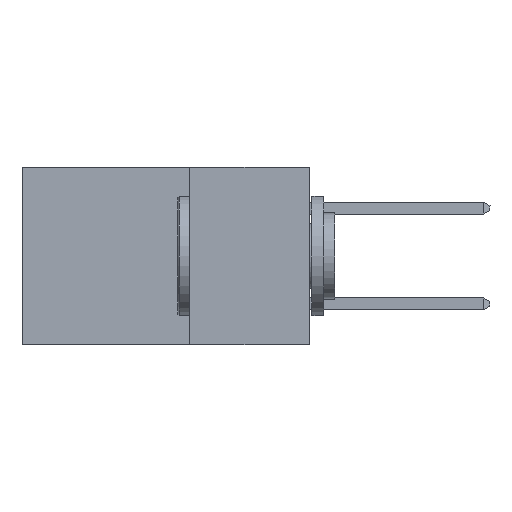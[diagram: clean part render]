
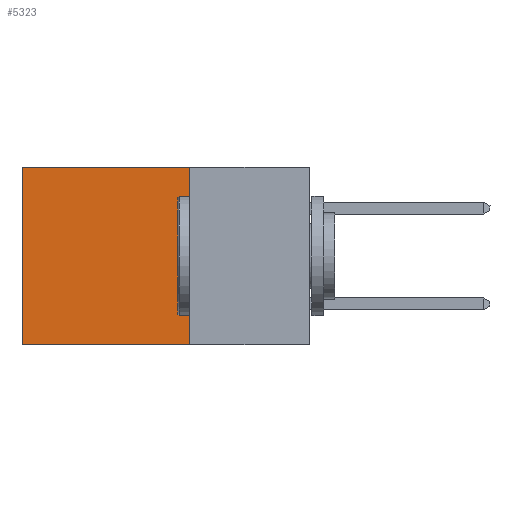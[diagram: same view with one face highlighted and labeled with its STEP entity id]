
A CAD part, left-side view. The second image highlights one B-rep face of the part: STEP entity #5323.
In plain terms, the highlighted planar face has unit normal (-1, 0, 0).
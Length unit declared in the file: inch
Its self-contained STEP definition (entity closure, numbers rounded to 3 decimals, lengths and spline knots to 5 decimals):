
#56 = EDGE_CURVE ( 'NONE', #404, #7802, #6104, .T. ) ;
#253 = CARTESIAN_POINT ( 'NONE',  ( 0.2875, 0.25, 0. ) ) ;
#404 = VERTEX_POINT ( 'NONE', #14413 ) ;
#565 = LINE ( 'NONE', #253, #7613 ) ;
#683 = ORIENTED_EDGE ( 'NONE', *, *, #14798, .F. ) ;
#1276 = DIRECTION ( 'NONE',  ( 0., 1., 0. ) ) ;
#1682 = ORIENTED_EDGE ( 'NONE', *, *, #11963, .F. ) ;
#1716 = DIRECTION ( 'NONE',  ( 0., 0., -1. ) ) ;
#1833 = VECTOR ( 'NONE', #8656, 39.37008 ) ;
#2574 = EDGE_CURVE ( 'NONE', #7402, #404, #11893, .T. ) ;
#3968 = CARTESIAN_POINT ( 'NONE',  ( 0.2875, 0.25, -0.37 ) ) ;
#4137 = CARTESIAN_POINT ( 'NONE',  ( 0.2875, 0.25, -0.37 ) ) ;
#5323 = ADVANCED_FACE ( 'NONE', ( #10335 ), #14903, .F. ) ;
#5620 = EDGE_LOOP ( 'NONE', ( #5697, #1682, #683, #10764 ) ) ;
#5697 = ORIENTED_EDGE ( 'NONE', *, *, #56, .T. ) ;
#5942 = VERTEX_POINT ( 'NONE', #4137 ) ;
#6104 = LINE ( 'NONE', #9427, #14824 ) ;
#6105 = CARTESIAN_POINT ( 'NONE',  ( 0.2875, 0.25, 0. ) ) ;
#6754 = DIRECTION ( 'NONE',  ( 0., 0., -1. ) ) ;
#7402 = VERTEX_POINT ( 'NONE', #6105 ) ;
#7613 = VECTOR ( 'NONE', #1716, 39.37008 ) ;
#7792 = CARTESIAN_POINT ( 'NONE',  ( 0.2875, 0.6, -0.37 ) ) ;
#7802 = VERTEX_POINT ( 'NONE', #7792 ) ;
#8387 = DIRECTION ( 'NONE',  ( 0., 0., -1. ) ) ;
#8656 = DIRECTION ( 'NONE',  ( 0., 1., 0. ) ) ;
#8833 = CARTESIAN_POINT ( 'NONE',  ( 0.2875, 0.25, 0. ) ) ;
#9427 = CARTESIAN_POINT ( 'NONE',  ( 0.2875, 0.6, 0. ) ) ;
#10328 = CARTESIAN_POINT ( 'NONE',  ( 0.2875, 0.25, 0. ) ) ;
#10335 = FACE_OUTER_BOUND ( 'NONE', #5620, .T. ) ;
#10764 = ORIENTED_EDGE ( 'NONE', *, *, #2574, .T. ) ;
#11481 = VECTOR ( 'NONE', #1276, 39.37008 ) ;
#11893 = LINE ( 'NONE', #8833, #1833 ) ;
#11963 = EDGE_CURVE ( 'NONE', #5942, #7802, #14529, .T. ) ;
#13870 = DIRECTION ( 'NONE',  ( 1., 0., 0. ) ) ;
#14413 = CARTESIAN_POINT ( 'NONE',  ( 0.2875, 0.6, 0. ) ) ;
#14529 = LINE ( 'NONE', #3968, #11481 ) ;
#14798 = EDGE_CURVE ( 'NONE', #7402, #5942, #565, .T. ) ;
#14814 = AXIS2_PLACEMENT_3D ( 'NONE', #10328, #13870, #6754 ) ;
#14824 = VECTOR ( 'NONE', #8387, 39.37008 ) ;
#14903 = PLANE ( 'NONE',  #14814 ) ;
